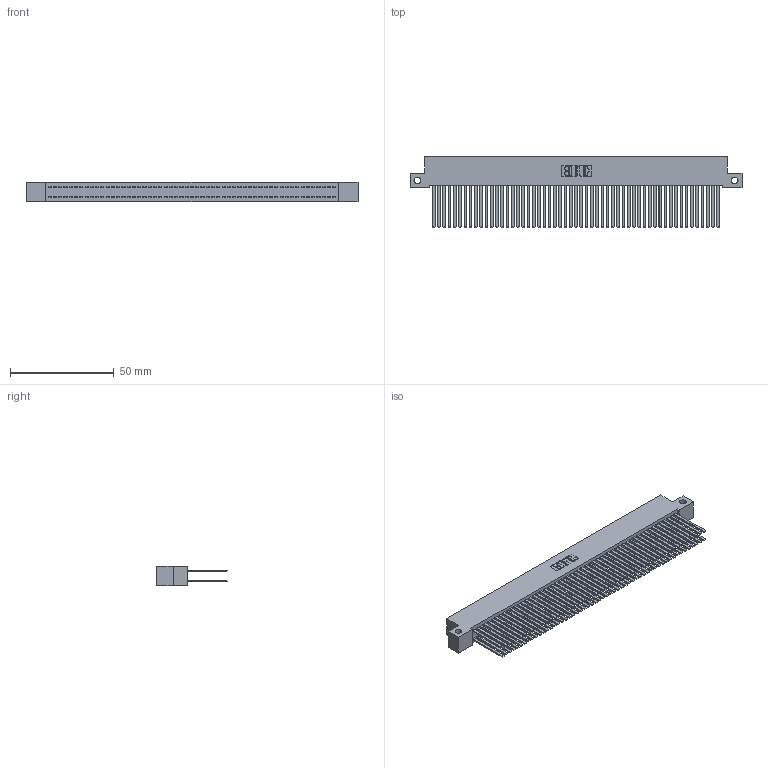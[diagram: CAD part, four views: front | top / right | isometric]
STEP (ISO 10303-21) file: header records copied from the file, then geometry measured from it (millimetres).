
FILE_DESCRIPTION (( 'STEP AP203' ), '1' );
FILE_NAME ('342-110-544-212.STEP', '2019-10-04T20:28:29', ( '' ), ( '' ), 'SwSTEP 2.0', 'SolidWorks 2016', '' );
FILE_SCHEMA (( 'CONFIG_CONTROL_DESIGN' ));
Length unit declared in the file: inch
Products named in the file (3): 342 Part_Side Mount; 345-292-001_345-293-144; 342-110-544-212
Assembly tree (111 placements, depth 2):
  342-110-544-212
    342 Part_Side Mount
    345-292-001_345-293-144  x110
Bounding box: 160.02 x 34.3 x 9.4 mm (x, y, z)
Volume: 15907.4 mm3; surface area: 30324.1 mm2
Topology: 111 solids, 111 shells, 5170 faces, 15369 edges, 10098 vertices
Faces by surface type: plane 3586, cylinder 1584
Entity records: 33389 total; most frequent: CARTESIAN_POINT 5514, ORIENTED_EDGE 5450, DIRECTION 4685, EDGE_CURVE 2725, LINE 2601, VECTOR 2601, VERTEX_POINT 1814, AXIS2_PLACEMENT_3D 1042
